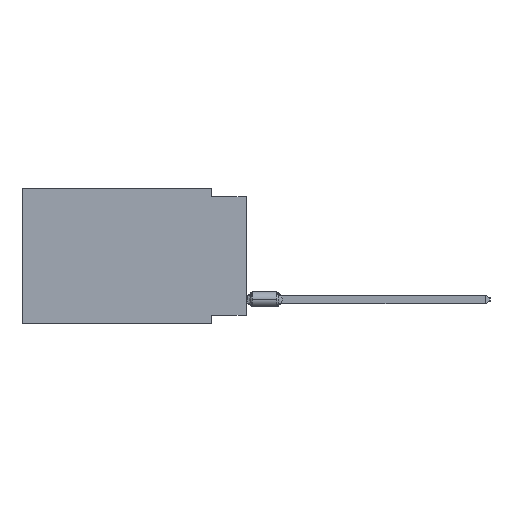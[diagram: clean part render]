
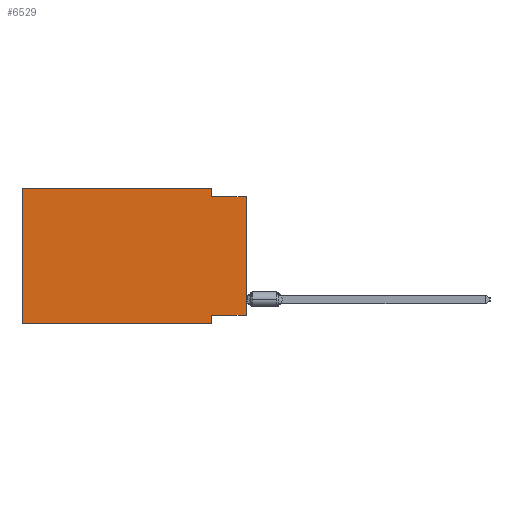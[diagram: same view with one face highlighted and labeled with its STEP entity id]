
A CAD part, left-side view. The second image highlights one B-rep face of the part: STEP entity #6529.
In plain terms, the highlighted planar face has unit normal (-1, 0, 0).
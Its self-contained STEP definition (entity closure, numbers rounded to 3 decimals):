
#262 = CARTESIAN_POINT ( 'NONE',  ( 0., 16.383, 0. ) ) ;
#1309 = LINE ( 'NONE', #42076, #35171 ) ;
#1320 = AXIS2_PLACEMENT_3D ( 'NONE', #18719, #7535, #38891 ) ;
#1366 = DIRECTION ( 'NONE',  ( 0., -1., 0. ) ) ;
#2561 = LINE ( 'NONE', #43337, #25038 ) ;
#2699 = ORIENTED_EDGE ( 'NONE', *, *, #11896, .F. ) ;
#3161 = VERTEX_POINT ( 'NONE', #39078 ) ;
#3998 = VERTEX_POINT ( 'NONE', #21723 ) ;
#4585 = ORIENTED_EDGE ( 'NONE', *, *, #14776, .F. ) ;
#6529 = ADVANCED_FACE ( 'NONE', ( #29013 ), #24994, .F. ) ;
#7250 = VECTOR ( 'NONE', #32975, 1000. ) ;
#7535 = DIRECTION ( 'NONE',  ( 1., 0., 0. ) ) ;
#7631 = LINE ( 'NONE', #21737, #7746 ) ;
#7746 = VECTOR ( 'NONE', #1366, 1000. ) ;
#8831 = VECTOR ( 'NONE', #27665, 1000. ) ;
#10043 = VECTOR ( 'NONE', #40803, 1000. ) ;
#10473 = VERTEX_POINT ( 'NONE', #23726 ) ;
#11589 = DIRECTION ( 'NONE',  ( 0., 0., -1. ) ) ;
#11896 = EDGE_CURVE ( 'NONE', #21351, #3161, #7631, .T. ) ;
#12409 = DIRECTION ( 'NONE',  ( 0., -1., 0. ) ) ;
#14111 = EDGE_CURVE ( 'NONE', #20874, #10473, #2561, .T. ) ;
#14776 = EDGE_CURVE ( 'NONE', #20874, #21351, #41681, .T. ) ;
#15013 = CARTESIAN_POINT ( 'NONE',  ( 0., 0., -0.635 ) ) ;
#16477 = CARTESIAN_POINT ( 'NONE',  ( 0., 16.383, -9.906 ) ) ;
#18719 = CARTESIAN_POINT ( 'NONE',  ( 0., 16.383, 0. ) ) ;
#20874 = VERTEX_POINT ( 'NONE', #16477 ) ;
#21020 = DIRECTION ( 'NONE',  ( 0., 1., 0. ) ) ;
#21239 = VECTOR ( 'NONE', #21968, 1000. ) ;
#21351 = VERTEX_POINT ( 'NONE', #37815 ) ;
#21723 = CARTESIAN_POINT ( 'NONE',  ( 0., 0., -9.271 ) ) ;
#21737 = CARTESIAN_POINT ( 'NONE',  ( 0., 16.383, 0. ) ) ;
#21853 = EDGE_LOOP ( 'NONE', ( #24149, #35999, #21954, #2699, #4585, #28441, #39595, #44138 ) ) ;
#21954 = ORIENTED_EDGE ( 'NONE', *, *, #31025, .F. ) ;
#21968 = DIRECTION ( 'NONE',  ( 0., -1., 0. ) ) ;
#23726 = CARTESIAN_POINT ( 'NONE',  ( 0., 2.54, -9.906 ) ) ;
#24149 = ORIENTED_EDGE ( 'NONE', *, *, #35107, .T. ) ;
#24456 = CARTESIAN_POINT ( 'NONE',  ( 0., 2.54, -9.271 ) ) ;
#24631 = VERTEX_POINT ( 'NONE', #24456 ) ;
#24994 = PLANE ( 'NONE',  #1320 ) ;
#25038 = VECTOR ( 'NONE', #12409, 1000. ) ;
#25878 = CARTESIAN_POINT ( 'NONE',  ( 0., 2.54, -0.635 ) ) ;
#26128 = EDGE_CURVE ( 'NONE', #38894, #35161, #42812, .T. ) ;
#27665 = DIRECTION ( 'NONE',  ( 0., 0., 1. ) ) ;
#27994 = VECTOR ( 'NONE', #11589, 1000. ) ;
#28441 = ORIENTED_EDGE ( 'NONE', *, *, #14111, .T. ) ;
#29013 = FACE_OUTER_BOUND ( 'NONE', #21853, .T. ) ;
#29161 = CARTESIAN_POINT ( 'NONE',  ( 0., 2.54, -9.906 ) ) ;
#31022 = CARTESIAN_POINT ( 'NONE',  ( 0., 0., 0. ) ) ;
#31025 = EDGE_CURVE ( 'NONE', #3161, #38894, #42977, .T. ) ;
#31908 = CARTESIAN_POINT ( 'NONE',  ( 0., 0., -0.635 ) ) ;
#32750 = LINE ( 'NONE', #29161, #7250 ) ;
#32975 = DIRECTION ( 'NONE',  ( 0., 0., -1. ) ) ;
#35107 = EDGE_CURVE ( 'NONE', #3998, #35161, #41349, .T. ) ;
#35161 = VERTEX_POINT ( 'NONE', #31908 ) ;
#35171 = VECTOR ( 'NONE', #21020, 1000. ) ;
#35999 = ORIENTED_EDGE ( 'NONE', *, *, #26128, .F. ) ;
#37160 = EDGE_CURVE ( 'NONE', #3998, #24631, #1309, .T. ) ;
#37815 = CARTESIAN_POINT ( 'NONE',  ( 0., 16.383, 0. ) ) ;
#38891 = DIRECTION ( 'NONE',  ( 0., 0., -1. ) ) ;
#38894 = VERTEX_POINT ( 'NONE', #25878 ) ;
#39078 = CARTESIAN_POINT ( 'NONE',  ( 0., 2.54, 0. ) ) ;
#39595 = ORIENTED_EDGE ( 'NONE', *, *, #44229, .F. ) ;
#39616 = CARTESIAN_POINT ( 'NONE',  ( 0., 2.54, 0. ) ) ;
#40803 = DIRECTION ( 'NONE',  ( 0., 0., 1. ) ) ;
#41349 = LINE ( 'NONE', #31022, #8831 ) ;
#41681 = LINE ( 'NONE', #262, #10043 ) ;
#42076 = CARTESIAN_POINT ( 'NONE',  ( 0., 0., -9.271 ) ) ;
#42812 = LINE ( 'NONE', #15013, #21239 ) ;
#42977 = LINE ( 'NONE', #39616, #27994 ) ;
#43337 = CARTESIAN_POINT ( 'NONE',  ( 0., 16.383, -9.906 ) ) ;
#44138 = ORIENTED_EDGE ( 'NONE', *, *, #37160, .F. ) ;
#44229 = EDGE_CURVE ( 'NONE', #24631, #10473, #32750, .T. ) ;
